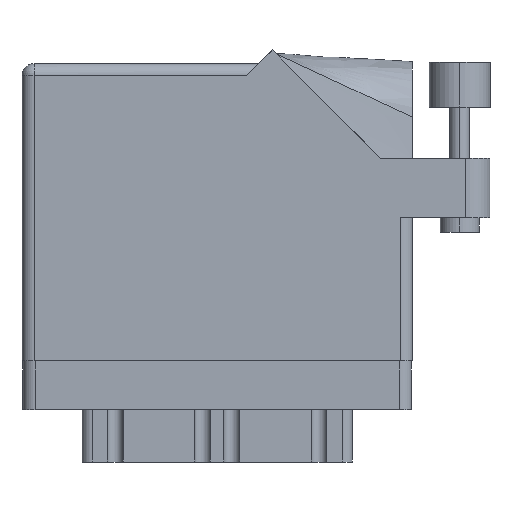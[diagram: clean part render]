
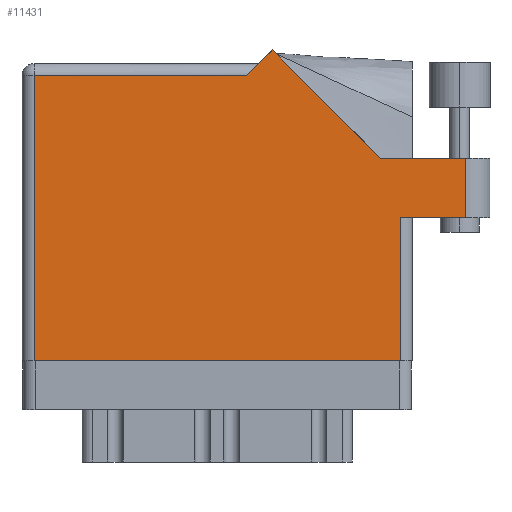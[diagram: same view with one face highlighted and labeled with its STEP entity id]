
A CAD part, front view. The second image highlights one B-rep face of the part: STEP entity #11431.
In plain terms, the highlighted face is planar.
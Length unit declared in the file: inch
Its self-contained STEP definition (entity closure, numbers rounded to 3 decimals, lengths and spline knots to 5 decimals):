
#588 = PLANE ( 'NONE',  #36527 ) ;
#920 = CARTESIAN_POINT ( 'NONE',  ( 2.01, 0.737, 0. ) ) ;
#983 = DIRECTION ( 'NONE',  ( -1., 0., 0. ) ) ;
#1118 = LINE ( 'NONE', #920, #20294 ) ;
#1774 = DIRECTION ( 'NONE',  ( -0.707, 0.707, 0. ) ) ;
#2106 = ORIENTED_EDGE ( 'NONE', *, *, #21421, .T. ) ;
#3197 = EDGE_CURVE ( 'NONE', #18500, #5239, #10970, .T. ) ;
#3500 = VERTEX_POINT ( 'NONE', #21507 ) ;
#3721 = CARTESIAN_POINT ( 'NONE',  ( 1.84442, 1.044, 0. ) ) ;
#4097 = CARTESIAN_POINT ( 'NONE',  ( 0., 1.468, 0. ) ) ;
#5239 = VERTEX_POINT ( 'NONE', #38624 ) ;
#6012 = ORIENTED_EDGE ( 'NONE', *, *, #25049, .T. ) ;
#6240 = VERTEX_POINT ( 'NONE', #19486 ) ;
#7385 = CARTESIAN_POINT ( 'NONE',  ( 2.285, 1.044, 0. ) ) ;
#8031 = CARTESIAN_POINT ( 'NONE',  ( 0.062, 0., 0. ) ) ;
#8442 = ORIENTED_EDGE ( 'NONE', *, *, #20751, .T. ) ;
#8760 = ORIENTED_EDGE ( 'NONE', *, *, #19397, .T. ) ;
#10208 = VERTEX_POINT ( 'NONE', #3721 ) ;
#10297 = CARTESIAN_POINT ( 'NONE',  ( 0.062, 1.468, 0. ) ) ;
#10970 = LINE ( 'NONE', #8031, #29126 ) ;
#11205 = VECTOR ( 'NONE', #1774, 39.37008 ) ;
#11431 = ADVANCED_FACE ( 'NONE', ( #22350 ), #588, .F. ) ;
#11946 = DIRECTION ( 'NONE',  ( -0.707, -0.707, 0. ) ) ;
#12112 = ORIENTED_EDGE ( 'NONE', *, *, #16587, .T. ) ;
#12911 = VERTEX_POINT ( 'NONE', #33330 ) ;
#12958 = DIRECTION ( 'NONE',  ( 0., 1., 0. ) ) ;
#13345 = CARTESIAN_POINT ( 'NONE',  ( 1.155, 1.468, 0. ) ) ;
#13725 = CARTESIAN_POINT ( 'NONE',  ( 1.84442, 1.044, 0. ) ) ;
#14639 = ORIENTED_EDGE ( 'NONE', *, *, #36255, .T. ) ;
#15823 = VERTEX_POINT ( 'NONE', #34500 ) ;
#15830 = LINE ( 'NONE', #30732, #17576 ) ;
#16587 = EDGE_CURVE ( 'NONE', #31164, #10208, #18772, .T. ) ;
#17576 = VECTOR ( 'NONE', #27813, 39.37008 ) ;
#17719 = VECTOR ( 'NONE', #34070, 39.37008 ) ;
#18500 = VERTEX_POINT ( 'NONE', #10297 ) ;
#18772 = LINE ( 'NONE', #30325, #28778 ) ;
#19205 = DIRECTION ( 'NONE',  ( 0., 0., -1. ) ) ;
#19397 = EDGE_CURVE ( 'NONE', #15823, #6240, #24730, .T. ) ;
#19486 = CARTESIAN_POINT ( 'NONE',  ( 1.948, 0.737, 0. ) ) ;
#19522 = DIRECTION ( 'NONE',  ( 0., 1., 0. ) ) ;
#19987 = DIRECTION ( 'NONE',  ( 0., -1., 0. ) ) ;
#20003 = LINE ( 'NONE', #13725, #11205 ) ;
#20294 = VECTOR ( 'NONE', #21904, 39.37008 ) ;
#20751 = EDGE_CURVE ( 'NONE', #12911, #30609, #36197, .T. ) ;
#21421 = EDGE_CURVE ( 'NONE', #3500, #31164, #37125, .T. ) ;
#21507 = CARTESIAN_POINT ( 'NONE',  ( 2.285, 0.737, 0. ) ) ;
#21904 = DIRECTION ( 'NONE',  ( 1., 0., 0. ) ) ;
#22137 = LINE ( 'NONE', #4097, #17719 ) ;
#22350 = FACE_OUTER_BOUND ( 'NONE', #32663, .T. ) ;
#22566 = EDGE_CURVE ( 'NONE', #6240, #3500, #1118, .T. ) ;
#23855 = ORIENTED_EDGE ( 'NONE', *, *, #3197, .T. ) ;
#24259 = ORIENTED_EDGE ( 'NONE', *, *, #22566, .T. ) ;
#24730 = LINE ( 'NONE', #30775, #35628 ) ;
#25049 = EDGE_CURVE ( 'NONE', #30609, #18500, #22137, .T. ) ;
#25228 = VECTOR ( 'NONE', #11946, 39.37008 ) ;
#27813 = DIRECTION ( 'NONE',  ( 1., 0., 0. ) ) ;
#28778 = VECTOR ( 'NONE', #30135, 39.37008 ) ;
#29126 = VECTOR ( 'NONE', #19987, 39.37008 ) ;
#29565 = EDGE_CURVE ( 'NONE', #10208, #12911, #20003, .T. ) ;
#30135 = DIRECTION ( 'NONE',  ( -1., 0., 0. ) ) ;
#30325 = CARTESIAN_POINT ( 'NONE',  ( 2.41, 1.044, 0. ) ) ;
#30609 = VERTEX_POINT ( 'NONE', #13345 ) ;
#30732 = CARTESIAN_POINT ( 'NONE',  ( 0., 0., 0. ) ) ;
#30775 = CARTESIAN_POINT ( 'NONE',  ( 1.948, 0.737, 0. ) ) ;
#31164 = VERTEX_POINT ( 'NONE', #38315 ) ;
#31500 = VECTOR ( 'NONE', #19522, 39.37008 ) ;
#32663 = EDGE_LOOP ( 'NONE', ( #24259, #2106, #12112, #34367, #8442, #6012, #23855, #14639, #8760 ) ) ;
#33330 = CARTESIAN_POINT ( 'NONE',  ( 1.28771, 1.60071, 0. ) ) ;
#34070 = DIRECTION ( 'NONE',  ( -1., 0., 0. ) ) ;
#34367 = ORIENTED_EDGE ( 'NONE', *, *, #29565, .T. ) ;
#34500 = CARTESIAN_POINT ( 'NONE',  ( 1.948, 0., 0. ) ) ;
#35628 = VECTOR ( 'NONE', #12958, 39.37008 ) ;
#35806 = CARTESIAN_POINT ( 'NONE',  ( 1.217, 1.53, 0. ) ) ;
#36197 = LINE ( 'NONE', #35806, #25228 ) ;
#36255 = EDGE_CURVE ( 'NONE', #5239, #15823, #15830, .T. ) ;
#36527 = AXIS2_PLACEMENT_3D ( 'NONE', #36615, #19205, #983 ) ;
#36615 = CARTESIAN_POINT ( 'NONE',  ( 0., 1.53, 0. ) ) ;
#37125 = LINE ( 'NONE', #7385, #31500 ) ;
#38315 = CARTESIAN_POINT ( 'NONE',  ( 2.285, 1.044, 0. ) ) ;
#38624 = CARTESIAN_POINT ( 'NONE',  ( 0.062, 0., 0. ) ) ;
